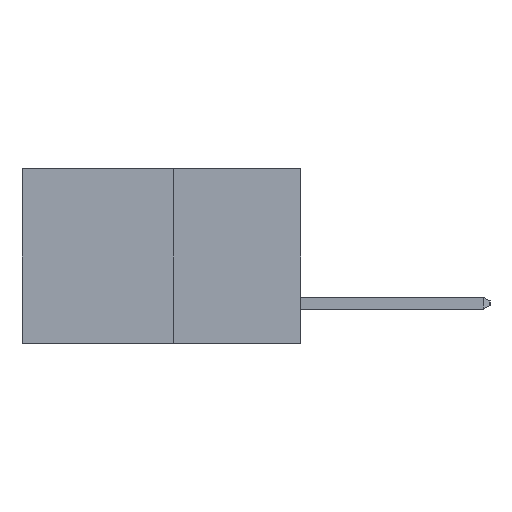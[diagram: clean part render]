
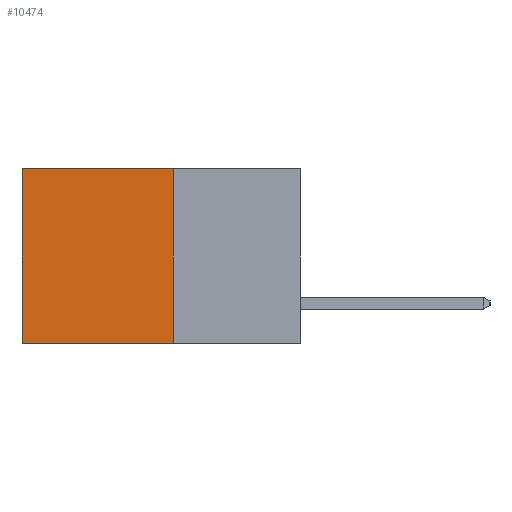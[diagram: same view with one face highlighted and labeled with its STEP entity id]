
A CAD part, left-side view. The second image highlights one B-rep face of the part: STEP entity #10474.
In plain terms, the highlighted planar face has unit normal (-1, 0, 0).
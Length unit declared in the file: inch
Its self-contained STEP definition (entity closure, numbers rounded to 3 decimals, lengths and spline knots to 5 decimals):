
#145 = ORIENTED_EDGE ( 'NONE', *, *, #7150, .F. ) ;
#407 = PLANE ( 'NONE',  #3323 ) ;
#593 = DIRECTION ( 'NONE',  ( 0., 1., 0. ) ) ;
#651 = ORIENTED_EDGE ( 'NONE', *, *, #8843, .F. ) ;
#820 = CARTESIAN_POINT ( 'NONE',  ( 0.277, 0.27, -0.37 ) ) ;
#850 = EDGE_CURVE ( 'NONE', #8447, #6245, #7029, .T. ) ;
#1988 = VECTOR ( 'NONE', #9819, 39.37008 ) ;
#2386 = DIRECTION ( 'NONE',  ( 1., 0., 0. ) ) ;
#2838 = CARTESIAN_POINT ( 'NONE',  ( 0.277, 0.27, 0. ) ) ;
#3053 = CARTESIAN_POINT ( 'NONE',  ( 0.277, 0.27, 0. ) ) ;
#3323 = AXIS2_PLACEMENT_3D ( 'NONE', #11772, #2386, #9014 ) ;
#3856 = EDGE_LOOP ( 'NONE', ( #11276, #651, #145, #7958 ) ) ;
#4103 = EDGE_CURVE ( 'NONE', #6245, #7116, #6688, .T. ) ;
#4184 = LINE ( 'NONE', #820, #4798 ) ;
#4445 = VECTOR ( 'NONE', #593, 39.37008 ) ;
#4798 = VECTOR ( 'NONE', #10308, 39.37008 ) ;
#6213 = FACE_OUTER_BOUND ( 'NONE', #3856, .T. ) ;
#6245 = VERTEX_POINT ( 'NONE', #8917 ) ;
#6366 = CARTESIAN_POINT ( 'NONE',  ( 0.277, 0.59, -0.37 ) ) ;
#6406 = VECTOR ( 'NONE', #10790, 39.37008 ) ;
#6688 = LINE ( 'NONE', #6366, #6406 ) ;
#6985 = LINE ( 'NONE', #7277, #4445 ) ;
#7029 = LINE ( 'NONE', #3053, #1988 ) ;
#7116 = VERTEX_POINT ( 'NONE', #8409 ) ;
#7150 = EDGE_CURVE ( 'NONE', #8447, #10871, #4184, .T. ) ;
#7277 = CARTESIAN_POINT ( 'NONE',  ( 0.277, 0.27, -0.37 ) ) ;
#7958 = ORIENTED_EDGE ( 'NONE', *, *, #850, .T. ) ;
#8409 = CARTESIAN_POINT ( 'NONE',  ( 0.277, 0.59, -0.37 ) ) ;
#8447 = VERTEX_POINT ( 'NONE', #2838 ) ;
#8843 = EDGE_CURVE ( 'NONE', #10871, #7116, #6985, .T. ) ;
#8917 = CARTESIAN_POINT ( 'NONE',  ( 0.277, 0.59, 0. ) ) ;
#9014 = DIRECTION ( 'NONE',  ( 0., 0., -1. ) ) ;
#9819 = DIRECTION ( 'NONE',  ( 0., 1., 0. ) ) ;
#10308 = DIRECTION ( 'NONE',  ( 0., 0., -1. ) ) ;
#10474 = ADVANCED_FACE ( 'NONE', ( #6213 ), #407, .F. ) ;
#10540 = CARTESIAN_POINT ( 'NONE',  ( 0.277, 0.27, -0.37 ) ) ;
#10790 = DIRECTION ( 'NONE',  ( 0., 0., -1. ) ) ;
#10871 = VERTEX_POINT ( 'NONE', #10540 ) ;
#11276 = ORIENTED_EDGE ( 'NONE', *, *, #4103, .T. ) ;
#11772 = CARTESIAN_POINT ( 'NONE',  ( 0.277, 0.27, -0.37 ) ) ;
